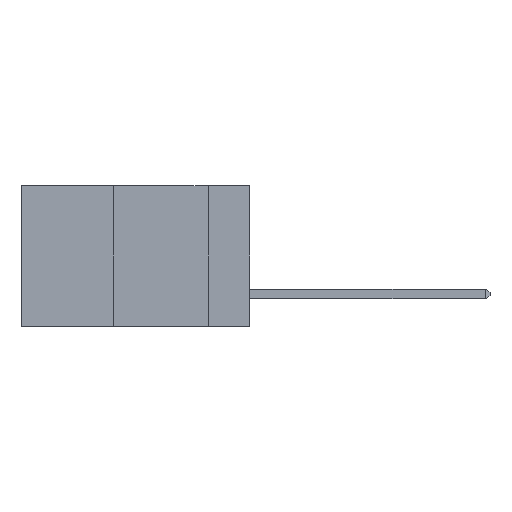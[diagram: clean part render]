
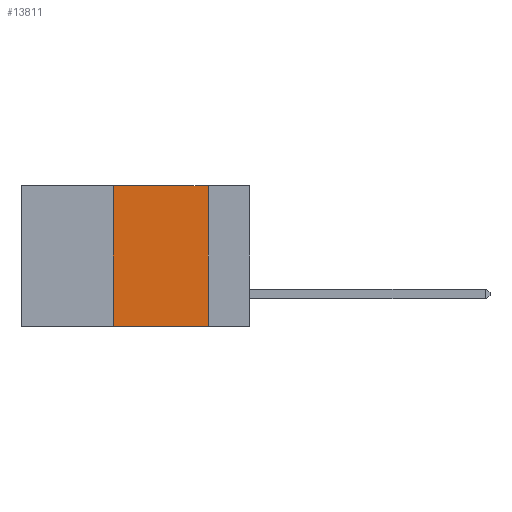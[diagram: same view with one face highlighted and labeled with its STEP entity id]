
A CAD part, left-side view. The second image highlights one B-rep face of the part: STEP entity #13811.
In plain terms, the highlighted planar face has unit normal (-1, 0, 0).
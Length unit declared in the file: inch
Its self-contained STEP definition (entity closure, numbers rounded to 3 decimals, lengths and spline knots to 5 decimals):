
#117 = CARTESIAN_POINT ( 'NONE',  ( 0., 0.11, 0. ) ) ;
#241 = EDGE_CURVE ( 'NONE', #20473, #12112, #2962, .T. ) ;
#669 = EDGE_LOOP ( 'NONE', ( #5966, #13233, #18537, #19766 ) ) ;
#826 = DIRECTION ( 'NONE',  ( 1., 0., 0. ) ) ;
#912 = CARTESIAN_POINT ( 'NONE',  ( 0., 0.36, 0. ) ) ;
#2962 = LINE ( 'NONE', #13274, #13190 ) ;
#3887 = CARTESIAN_POINT ( 'NONE',  ( 0., 0.36, 0. ) ) ;
#4265 = AXIS2_PLACEMENT_3D ( 'NONE', #9243, #826, #15189 ) ;
#4804 = VECTOR ( 'NONE', #14557, 39.37008 ) ;
#4831 = VERTEX_POINT ( 'NONE', #7259 ) ;
#5289 = FACE_OUTER_BOUND ( 'NONE', #669, .T. ) ;
#5966 = ORIENTED_EDGE ( 'NONE', *, *, #18977, .F. ) ;
#5982 = DIRECTION ( 'NONE',  ( 0., 0., 1. ) ) ;
#6009 = EDGE_CURVE ( 'NONE', #11234, #20473, #14749, .T. ) ;
#6420 = VECTOR ( 'NONE', #22911, 39.37008 ) ;
#7017 = CARTESIAN_POINT ( 'NONE',  ( 0., 0.6, -0.37 ) ) ;
#7259 = CARTESIAN_POINT ( 'NONE',  ( 0., 0.11, -0.37 ) ) ;
#8284 = CARTESIAN_POINT ( 'NONE',  ( 0., 0.36, -0.37 ) ) ;
#9243 = CARTESIAN_POINT ( 'NONE',  ( 0., 0.6, 0. ) ) ;
#9493 = CARTESIAN_POINT ( 'NONE',  ( 0., 0.11, 0. ) ) ;
#11234 = VERTEX_POINT ( 'NONE', #8284 ) ;
#11459 = EDGE_CURVE ( 'NONE', #11234, #4831, #17725, .T. ) ;
#12112 = VERTEX_POINT ( 'NONE', #9493 ) ;
#13190 = VECTOR ( 'NONE', #13250, 39.37008 ) ;
#13233 = ORIENTED_EDGE ( 'NONE', *, *, #241, .F. ) ;
#13250 = DIRECTION ( 'NONE',  ( 0., -1., 0. ) ) ;
#13274 = CARTESIAN_POINT ( 'NONE',  ( 0., 0.6, 0. ) ) ;
#13811 = ADVANCED_FACE ( 'NONE', ( #5289 ), #23067, .F. ) ;
#14557 = DIRECTION ( 'NONE',  ( 0., 0., -1. ) ) ;
#14749 = LINE ( 'NONE', #3887, #25256 ) ;
#15189 = DIRECTION ( 'NONE',  ( 0., 0., -1. ) ) ;
#17725 = LINE ( 'NONE', #7017, #6420 ) ;
#18537 = ORIENTED_EDGE ( 'NONE', *, *, #6009, .F. ) ;
#18977 = EDGE_CURVE ( 'NONE', #12112, #4831, #20226, .T. ) ;
#19766 = ORIENTED_EDGE ( 'NONE', *, *, #11459, .T. ) ;
#20226 = LINE ( 'NONE', #117, #4804 ) ;
#20473 = VERTEX_POINT ( 'NONE', #912 ) ;
#22911 = DIRECTION ( 'NONE',  ( 0., -1., 0. ) ) ;
#23067 = PLANE ( 'NONE',  #4265 ) ;
#25256 = VECTOR ( 'NONE', #5982, 39.37008 ) ;
